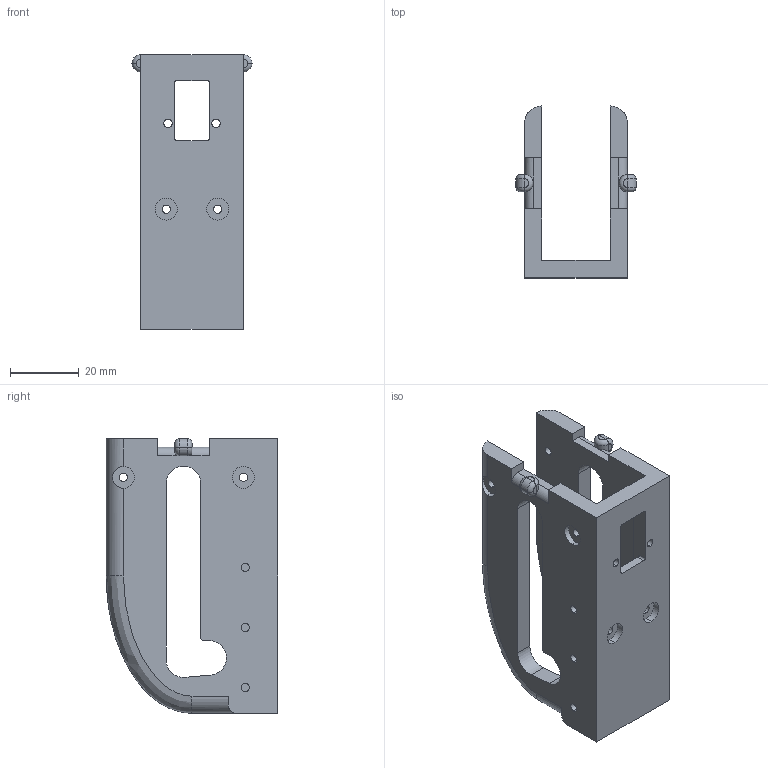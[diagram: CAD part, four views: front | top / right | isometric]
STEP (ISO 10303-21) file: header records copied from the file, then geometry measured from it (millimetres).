
FILE_DESCRIPTION (( 'STEP AP203' ), '1' );
FILE_NAME ('Body.STEP', '2013-11-14T05:07:17', ( '' ), ( '' ), 'SwSTEP 2.0', 'SolidWorks 2013', '' );
FILE_SCHEMA (( 'CONFIG_CONTROL_DESIGN' ));
Length unit declared in the file: millimetre
Products named in the file (1): Body
Bounding box: 35 x 50 x 80 mm (x, y, z)
Volume: 35269.6 mm3; surface area: 19121.4 mm2
Topology: 1 solids, 1 shells, 125 faces, 328 edges, 209 vertices
Faces by surface type: cylinder 67, plane 44, torus 12, bspline 2
Entity records: 4426 total; most frequent: CARTESIAN_POINT 1133, DIRECTION 699, ORIENTED_EDGE 656, EDGE_CURVE 328, AXIS2_PLACEMENT_3D 267, VERTEX_POINT 209, LINE 165, VECTOR 165
